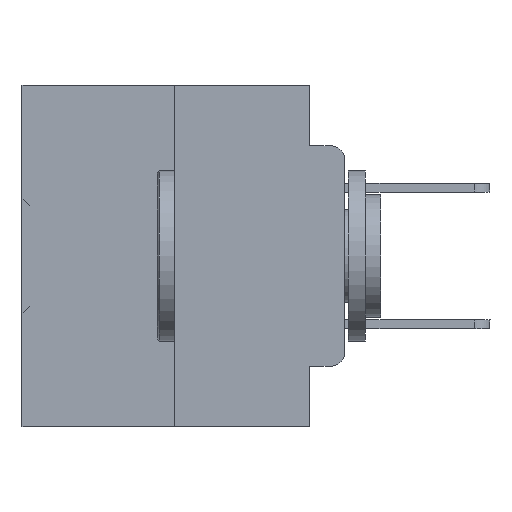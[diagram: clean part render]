
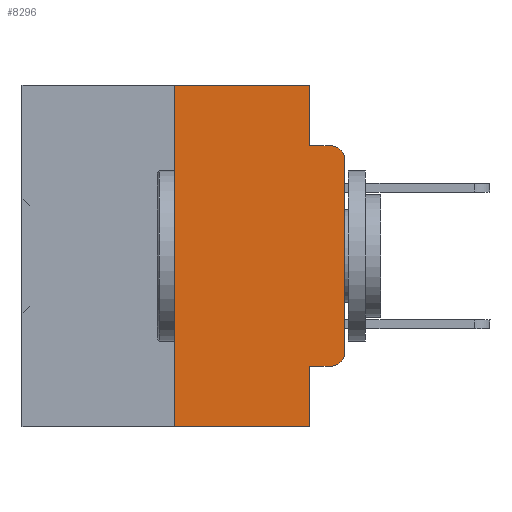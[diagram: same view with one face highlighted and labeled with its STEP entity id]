
A CAD part, left-side view. The second image highlights one B-rep face of the part: STEP entity #8296.
In plain terms, the highlighted planar face has unit normal (-1, 0, 0).
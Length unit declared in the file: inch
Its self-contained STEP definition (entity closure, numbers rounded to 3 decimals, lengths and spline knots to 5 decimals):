
#259 = CARTESIAN_POINT ( 'NONE',  ( 0., 0.25, 0. ) ) ;
#1034 = ORIENTED_EDGE ( 'NONE', *, *, #9378, .T. ) ;
#1144 = CARTESIAN_POINT ( 'NONE',  ( 0., 0.473, -0.5 ) ) ;
#1635 = VECTOR ( 'NONE', #19701, 39.37008 ) ;
#1920 = CARTESIAN_POINT ( 'NONE',  ( 0., 0.02, -0.3915 ) ) ;
#2236 = CARTESIAN_POINT ( 'NONE',  ( 0., 0., -0.1085 ) ) ;
#2359 = ORIENTED_EDGE ( 'NONE', *, *, #21038, .F. ) ;
#2861 = CARTESIAN_POINT ( 'NONE',  ( 0., 0.02, -0.0885 ) ) ;
#2898 = DIRECTION ( 'NONE',  ( 0., 0., -1. ) ) ;
#2910 = DIRECTION ( 'NONE',  ( -1., 0., 0. ) ) ;
#3677 = CIRCLE ( 'NONE', #36609, 0.02 ) ;
#4031 = AXIS2_PLACEMENT_3D ( 'NONE', #34020, #2910, #12371 ) ;
#4797 = LINE ( 'NONE', #8015, #17348 ) ;
#5725 = LINE ( 'NONE', #5901, #8220 ) ;
#5821 = ORIENTED_EDGE ( 'NONE', *, *, #25930, .T. ) ;
#5901 = CARTESIAN_POINT ( 'NONE',  ( 0., 0.473, 0. ) ) ;
#6711 = CARTESIAN_POINT ( 'NONE',  ( 0., 0.051, 0. ) ) ;
#6936 = EDGE_CURVE ( 'NONE', #21287, #15862, #36849, .T. ) ;
#8015 = CARTESIAN_POINT ( 'NONE',  ( 0., 0.051, 0. ) ) ;
#8171 = ORIENTED_EDGE ( 'NONE', *, *, #11058, .T. ) ;
#8220 = VECTOR ( 'NONE', #21035, 39.37008 ) ;
#8296 = ADVANCED_FACE ( 'NONE', ( #32361 ), #26069, .F. ) ;
#8519 = VERTEX_POINT ( 'NONE', #39645 ) ;
#9147 = DIRECTION ( 'NONE',  ( 0., 0., 1. ) ) ;
#9378 = EDGE_CURVE ( 'NONE', #36730, #18205, #10430, .T. ) ;
#9951 = LINE ( 'NONE', #22256, #17573 ) ;
#10430 = LINE ( 'NONE', #22726, #1635 ) ;
#11058 = EDGE_CURVE ( 'NONE', #18205, #12576, #3677, .T. ) ;
#12209 = VERTEX_POINT ( 'NONE', #39751 ) ;
#12371 = DIRECTION ( 'NONE',  ( 0., 0., -1. ) ) ;
#12540 = EDGE_CURVE ( 'NONE', #32621, #29463, #38892, .T. ) ;
#12576 = VERTEX_POINT ( 'NONE', #18825 ) ;
#12710 = EDGE_CURVE ( 'NONE', #12209, #29463, #9951, .T. ) ;
#13145 = VECTOR ( 'NONE', #2898, 39.37008 ) ;
#14012 = DIRECTION ( 'NONE',  ( 0., 0., -1. ) ) ;
#15735 = VECTOR ( 'NONE', #9147, 39.37008 ) ;
#15862 = VERTEX_POINT ( 'NONE', #19330 ) ;
#16075 = VECTOR ( 'NONE', #31437, 39.37008 ) ;
#16188 = EDGE_LOOP ( 'NONE', ( #25767, #24890, #20646, #31971, #2359, #21912, #5821, #24904, #1034, #8171 ) ) ;
#17196 = DIRECTION ( 'NONE',  ( 0., 0., -1. ) ) ;
#17247 = DIRECTION ( 'NONE',  ( -1., 0., 0. ) ) ;
#17348 = VECTOR ( 'NONE', #23340, 39.37008 ) ;
#17573 = VECTOR ( 'NONE', #25685, 39.37008 ) ;
#17770 = AXIS2_PLACEMENT_3D ( 'NONE', #19814, #38436, #17196 ) ;
#17961 = CARTESIAN_POINT ( 'NONE',  ( 0., 0.02, -0.4115 ) ) ;
#18205 = VERTEX_POINT ( 'NONE', #17961 ) ;
#18825 = CARTESIAN_POINT ( 'NONE',  ( 0., 0., -0.3915 ) ) ;
#19330 = CARTESIAN_POINT ( 'NONE',  ( 0., 0.25, 0. ) ) ;
#19483 = DIRECTION ( 'NONE',  ( 0., -1., 0. ) ) ;
#19701 = DIRECTION ( 'NONE',  ( 0., -1., 0. ) ) ;
#19814 = CARTESIAN_POINT ( 'NONE',  ( 0., 0.473, 0. ) ) ;
#20646 = ORIENTED_EDGE ( 'NONE', *, *, #12710, .F. ) ;
#21035 = DIRECTION ( 'NONE',  ( 0., -1., 0. ) ) ;
#21038 = EDGE_CURVE ( 'NONE', #15862, #38022, #5725, .T. ) ;
#21287 = VERTEX_POINT ( 'NONE', #25255 ) ;
#21330 = VECTOR ( 'NONE', #19483, 39.37008 ) ;
#21508 = CARTESIAN_POINT ( 'NONE',  ( 0., 0., 0. ) ) ;
#21912 = ORIENTED_EDGE ( 'NONE', *, *, #6936, .F. ) ;
#22102 = LINE ( 'NONE', #21508, #16075 ) ;
#22256 = CARTESIAN_POINT ( 'NONE',  ( 0., 0.051, -0.0885 ) ) ;
#22322 = LINE ( 'NONE', #1144, #21330 ) ;
#22726 = CARTESIAN_POINT ( 'NONE',  ( 0., 0.051, -0.4115 ) ) ;
#22966 = EDGE_CURVE ( 'NONE', #36730, #8519, #4797, .T. ) ;
#23340 = DIRECTION ( 'NONE',  ( 0., 0., -1. ) ) ;
#24890 = ORIENTED_EDGE ( 'NONE', *, *, #12540, .T. ) ;
#24904 = ORIENTED_EDGE ( 'NONE', *, *, #22966, .F. ) ;
#25255 = CARTESIAN_POINT ( 'NONE',  ( 0., 0.25, -0.5 ) ) ;
#25685 = DIRECTION ( 'NONE',  ( 0., -1., 0. ) ) ;
#25767 = ORIENTED_EDGE ( 'NONE', *, *, #36365, .T. ) ;
#25930 = EDGE_CURVE ( 'NONE', #21287, #8519, #22322, .T. ) ;
#26069 = PLANE ( 'NONE',  #17770 ) ;
#27756 = EDGE_CURVE ( 'NONE', #38022, #12209, #34400, .T. ) ;
#28130 = CARTESIAN_POINT ( 'NONE',  ( 0., 0.051, 0. ) ) ;
#29463 = VERTEX_POINT ( 'NONE', #2861 ) ;
#31437 = DIRECTION ( 'NONE',  ( 0., 0., 1. ) ) ;
#31971 = ORIENTED_EDGE ( 'NONE', *, *, #27756, .F. ) ;
#32361 = FACE_OUTER_BOUND ( 'NONE', #16188, .T. ) ;
#32621 = VERTEX_POINT ( 'NONE', #2236 ) ;
#34020 = CARTESIAN_POINT ( 'NONE',  ( 0., 0.02, -0.1085 ) ) ;
#34400 = LINE ( 'NONE', #6711, #13145 ) ;
#36365 = EDGE_CURVE ( 'NONE', #12576, #32621, #22102, .T. ) ;
#36609 = AXIS2_PLACEMENT_3D ( 'NONE', #1920, #17247, #14012 ) ;
#36730 = VERTEX_POINT ( 'NONE', #37206 ) ;
#36849 = LINE ( 'NONE', #259, #15735 ) ;
#37206 = CARTESIAN_POINT ( 'NONE',  ( 0., 0.051, -0.4115 ) ) ;
#38022 = VERTEX_POINT ( 'NONE', #28130 ) ;
#38436 = DIRECTION ( 'NONE',  ( 1., 0., 0. ) ) ;
#38892 = CIRCLE ( 'NONE', #4031, 0.02 ) ;
#39645 = CARTESIAN_POINT ( 'NONE',  ( 0., 0.051, -0.5 ) ) ;
#39751 = CARTESIAN_POINT ( 'NONE',  ( 0., 0.051, -0.0885 ) ) ;
